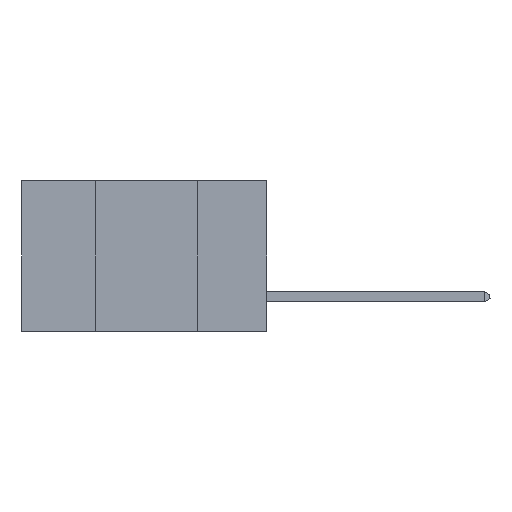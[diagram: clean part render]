
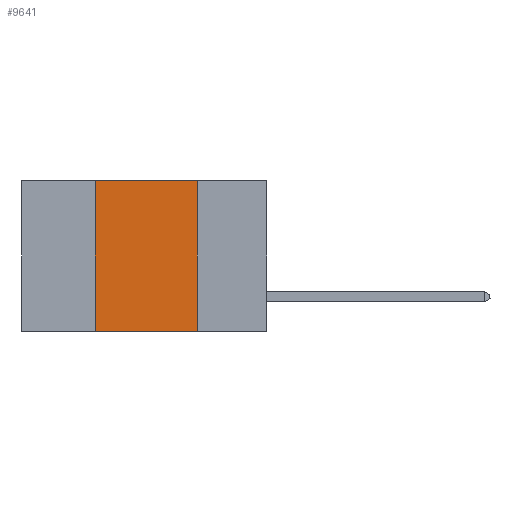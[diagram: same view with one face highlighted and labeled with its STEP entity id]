
A CAD part, left-side view. The second image highlights one B-rep face of the part: STEP entity #9641.
In plain terms, the highlighted planar face has unit normal (-1, 0, 0).
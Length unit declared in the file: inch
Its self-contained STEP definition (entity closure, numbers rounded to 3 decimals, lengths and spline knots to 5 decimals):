
#507 = DIRECTION ( 'NONE',  ( 0., 0., -1. ) ) ;
#760 = CARTESIAN_POINT ( 'NONE',  ( 0., 0.42, 0. ) ) ;
#1900 = EDGE_CURVE ( 'NONE', #21184, #22089, #22688, .T. ) ;
#2446 = EDGE_CURVE ( 'NONE', #22089, #10591, #10665, .T. ) ;
#3203 = DIRECTION ( 'NONE',  ( 0., -1., 0. ) ) ;
#3675 = LINE ( 'NONE', #24058, #19253 ) ;
#4083 = DIRECTION ( 'NONE',  ( 1., 0., 0. ) ) ;
#5049 = AXIS2_PLACEMENT_3D ( 'NONE', #19104, #4083, #507 ) ;
#5240 = LINE ( 'NONE', #19460, #16407 ) ;
#5643 = VECTOR ( 'NONE', #3203, 39.37008 ) ;
#5983 = CARTESIAN_POINT ( 'NONE',  ( 0., 0.42, 0. ) ) ;
#6818 = FACE_OUTER_BOUND ( 'NONE', #21657, .T. ) ;
#7041 = ORIENTED_EDGE ( 'NONE', *, *, #1900, .F. ) ;
#8885 = CARTESIAN_POINT ( 'NONE',  ( 0., 0.17, -0.37 ) ) ;
#9641 = ADVANCED_FACE ( 'NONE', ( #6818 ), #17377, .F. ) ;
#10591 = VERTEX_POINT ( 'NONE', #13275 ) ;
#10665 = LINE ( 'NONE', #18299, #5643 ) ;
#10690 = VECTOR ( 'NONE', #11449, 39.37008 ) ;
#11298 = ORIENTED_EDGE ( 'NONE', *, *, #13423, .T. ) ;
#11449 = DIRECTION ( 'NONE',  ( 0., 0., 1. ) ) ;
#12873 = DIRECTION ( 'NONE',  ( 0., -1., 0. ) ) ;
#13275 = CARTESIAN_POINT ( 'NONE',  ( 0., 0.17, 0. ) ) ;
#13423 = EDGE_CURVE ( 'NONE', #21184, #17932, #3675, .T. ) ;
#13715 = ORIENTED_EDGE ( 'NONE', *, *, #22558, .F. ) ;
#14846 = ORIENTED_EDGE ( 'NONE', *, *, #2446, .F. ) ;
#16407 = VECTOR ( 'NONE', #19117, 39.37008 ) ;
#17377 = PLANE ( 'NONE',  #5049 ) ;
#17932 = VERTEX_POINT ( 'NONE', #8885 ) ;
#18299 = CARTESIAN_POINT ( 'NONE',  ( 0., 0.6, 0. ) ) ;
#18479 = CARTESIAN_POINT ( 'NONE',  ( 0., 0.42, -0.37 ) ) ;
#19104 = CARTESIAN_POINT ( 'NONE',  ( 0., 0.6, 0. ) ) ;
#19117 = DIRECTION ( 'NONE',  ( 0., 0., -1. ) ) ;
#19253 = VECTOR ( 'NONE', #12873, 39.37008 ) ;
#19460 = CARTESIAN_POINT ( 'NONE',  ( 0., 0.17, 0. ) ) ;
#21184 = VERTEX_POINT ( 'NONE', #18479 ) ;
#21657 = EDGE_LOOP ( 'NONE', ( #13715, #14846, #7041, #11298 ) ) ;
#22089 = VERTEX_POINT ( 'NONE', #760 ) ;
#22558 = EDGE_CURVE ( 'NONE', #10591, #17932, #5240, .T. ) ;
#22688 = LINE ( 'NONE', #5983, #10690 ) ;
#24058 = CARTESIAN_POINT ( 'NONE',  ( 0., 0.6, -0.37 ) ) ;
